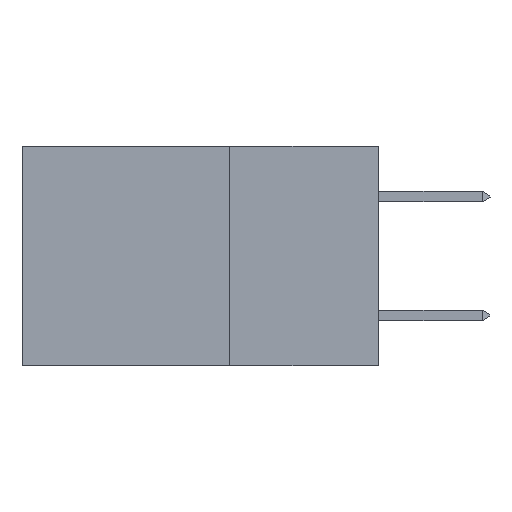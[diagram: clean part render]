
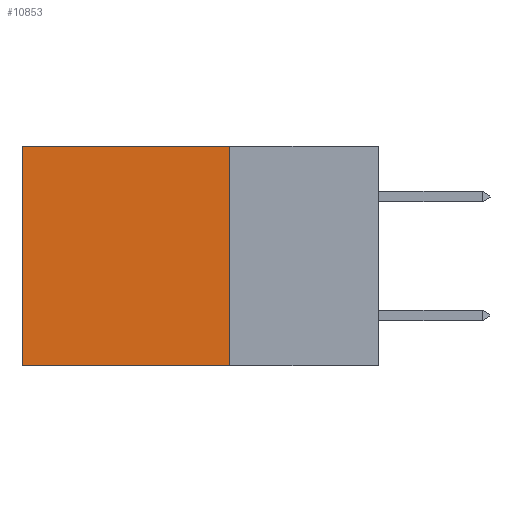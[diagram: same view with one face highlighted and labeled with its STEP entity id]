
A CAD part, left-side view. The second image highlights one B-rep face of the part: STEP entity #10853.
In plain terms, the highlighted planar face has unit normal (-1, 0, 0).
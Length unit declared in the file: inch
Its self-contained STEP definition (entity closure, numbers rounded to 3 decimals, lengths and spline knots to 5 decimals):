
#604 = VECTOR ( 'NONE', #6408, 39.37008 ) ;
#927 = DIRECTION ( 'NONE',  ( 0., 1., 0. ) ) ;
#1094 = CARTESIAN_POINT ( 'NONE',  ( 0.298, 0.25, 0. ) ) ;
#1291 = EDGE_CURVE ( 'NONE', #1620, #4130, #12570, .T. ) ;
#1394 = ORIENTED_EDGE ( 'NONE', *, *, #1291, .F. ) ;
#1494 = VERTEX_POINT ( 'NONE', #1594 ) ;
#1594 = CARTESIAN_POINT ( 'NONE',  ( 0.298, 0.6, -0.37 ) ) ;
#1620 = VERTEX_POINT ( 'NONE', #1094 ) ;
#2627 = VECTOR ( 'NONE', #927, 39.37008 ) ;
#2788 = ORIENTED_EDGE ( 'NONE', *, *, #12479, .F. ) ;
#3330 = AXIS2_PLACEMENT_3D ( 'NONE', #12683, #6595, #6734 ) ;
#3667 = PLANE ( 'NONE',  #3330 ) ;
#3894 = CARTESIAN_POINT ( 'NONE',  ( 0.298, 0.25, -0.37 ) ) ;
#3906 = DIRECTION ( 'NONE',  ( 0., 0., -1. ) ) ;
#4091 = CARTESIAN_POINT ( 'NONE',  ( 0.298, 0.6, 0. ) ) ;
#4130 = VERTEX_POINT ( 'NONE', #7801 ) ;
#4840 = VERTEX_POINT ( 'NONE', #4091 ) ;
#5539 = CARTESIAN_POINT ( 'NONE',  ( 0.298, 0.25, 0. ) ) ;
#5638 = LINE ( 'NONE', #7941, #6144 ) ;
#6144 = VECTOR ( 'NONE', #3906, 39.37008 ) ;
#6408 = DIRECTION ( 'NONE',  ( 0., 1., 0. ) ) ;
#6595 = DIRECTION ( 'NONE',  ( 1., 0., 0. ) ) ;
#6734 = DIRECTION ( 'NONE',  ( 0., 0., -1. ) ) ;
#6963 = LINE ( 'NONE', #3894, #2627 ) ;
#7430 = ORIENTED_EDGE ( 'NONE', *, *, #9276, .T. ) ;
#7801 = CARTESIAN_POINT ( 'NONE',  ( 0.298, 0.25, -0.37 ) ) ;
#7941 = CARTESIAN_POINT ( 'NONE',  ( 0.298, 0.6, 0. ) ) ;
#7946 = FACE_OUTER_BOUND ( 'NONE', #12787, .T. ) ;
#9276 = EDGE_CURVE ( 'NONE', #4840, #1494, #5638, .T. ) ;
#9601 = CARTESIAN_POINT ( 'NONE',  ( 0.298, 0.25, 0. ) ) ;
#10026 = VECTOR ( 'NONE', #11736, 39.37008 ) ;
#10072 = EDGE_CURVE ( 'NONE', #1620, #4840, #10521, .T. ) ;
#10521 = LINE ( 'NONE', #9601, #604 ) ;
#10853 = ADVANCED_FACE ( 'NONE', ( #7946 ), #3667, .F. ) ;
#11736 = DIRECTION ( 'NONE',  ( 0., 0., -1. ) ) ;
#11930 = ORIENTED_EDGE ( 'NONE', *, *, #10072, .T. ) ;
#12479 = EDGE_CURVE ( 'NONE', #4130, #1494, #6963, .T. ) ;
#12570 = LINE ( 'NONE', #5539, #10026 ) ;
#12683 = CARTESIAN_POINT ( 'NONE',  ( 0.298, 0.25, 0. ) ) ;
#12787 = EDGE_LOOP ( 'NONE', ( #7430, #2788, #1394, #11930 ) ) ;
